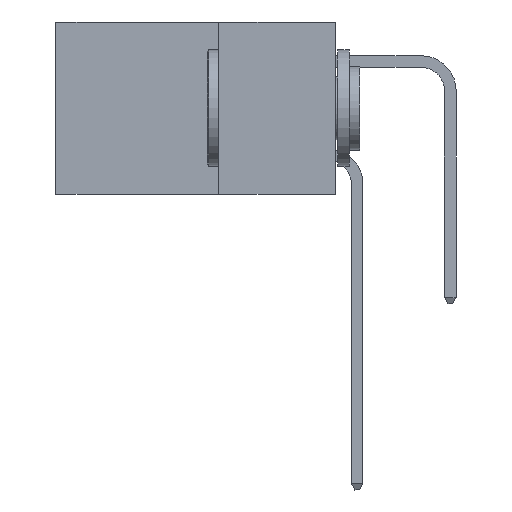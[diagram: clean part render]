
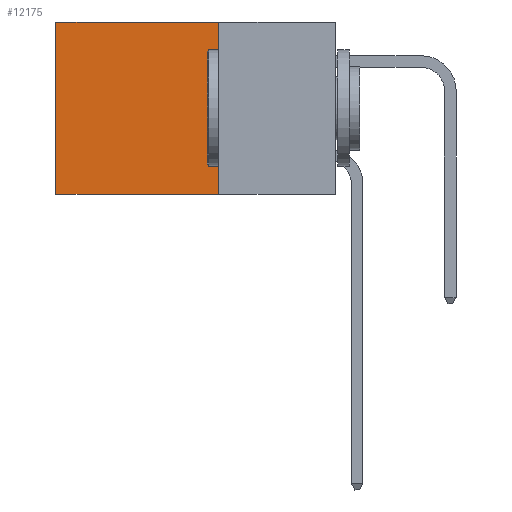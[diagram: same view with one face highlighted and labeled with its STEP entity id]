
A CAD part, left-side view. The second image highlights one B-rep face of the part: STEP entity #12175.
In plain terms, the highlighted planar face has unit normal (-1, 0, 0).
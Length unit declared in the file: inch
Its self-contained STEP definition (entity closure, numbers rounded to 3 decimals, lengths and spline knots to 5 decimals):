
#301 = VECTOR ( 'NONE', #4368, 39.37008 ) ;
#489 = VERTEX_POINT ( 'NONE', #13415 ) ;
#593 = VERTEX_POINT ( 'NONE', #12714 ) ;
#670 = FACE_OUTER_BOUND ( 'NONE', #8879, .T. ) ;
#791 = CARTESIAN_POINT ( 'NONE',  ( 0.2875, 0.25, -0.37 ) ) ;
#1101 = CARTESIAN_POINT ( 'NONE',  ( 0.2875, 0.25, 0. ) ) ;
#2113 = ORIENTED_EDGE ( 'NONE', *, *, #2717, .F. ) ;
#2717 = EDGE_CURVE ( 'NONE', #12955, #593, #13795, .T. ) ;
#2786 = DIRECTION ( 'NONE',  ( 1., 0., 0. ) ) ;
#3747 = LINE ( 'NONE', #8854, #6549 ) ;
#4368 = DIRECTION ( 'NONE',  ( 0., 1., 0. ) ) ;
#4374 = CARTESIAN_POINT ( 'NONE',  ( 0.2875, 0.25, -0.37 ) ) ;
#4686 = LINE ( 'NONE', #13721, #7107 ) ;
#4721 = VECTOR ( 'NONE', #8616, 39.37008 ) ;
#5503 = DIRECTION ( 'NONE',  ( 0., 0., -1. ) ) ;
#5987 = CARTESIAN_POINT ( 'NONE',  ( 0.2875, 0.25, 0. ) ) ;
#6377 = ORIENTED_EDGE ( 'NONE', *, *, #12557, .T. ) ;
#6549 = VECTOR ( 'NONE', #6787, 39.37008 ) ;
#6787 = DIRECTION ( 'NONE',  ( 0., 0., -1. ) ) ;
#7107 = VECTOR ( 'NONE', #5503, 39.37008 ) ;
#8616 = DIRECTION ( 'NONE',  ( 0., 1., 0. ) ) ;
#8854 = CARTESIAN_POINT ( 'NONE',  ( 0.2875, 0.6, 0. ) ) ;
#8858 = EDGE_CURVE ( 'NONE', #11644, #489, #9550, .T. ) ;
#8879 = EDGE_LOOP ( 'NONE', ( #6377, #2113, #11048, #10241 ) ) ;
#9550 = LINE ( 'NONE', #1101, #4721 ) ;
#10119 = DIRECTION ( 'NONE',  ( 0., 0., -1. ) ) ;
#10134 = EDGE_CURVE ( 'NONE', #11644, #12955, #4686, .T. ) ;
#10241 = ORIENTED_EDGE ( 'NONE', *, *, #8858, .T. ) ;
#11048 = ORIENTED_EDGE ( 'NONE', *, *, #10134, .F. ) ;
#11081 = PLANE ( 'NONE',  #13738 ) ;
#11644 = VERTEX_POINT ( 'NONE', #13297 ) ;
#12175 = ADVANCED_FACE ( 'NONE', ( #670 ), #11081, .F. ) ;
#12557 = EDGE_CURVE ( 'NONE', #489, #593, #3747, .T. ) ;
#12714 = CARTESIAN_POINT ( 'NONE',  ( 0.2875, 0.6, -0.37 ) ) ;
#12955 = VERTEX_POINT ( 'NONE', #791 ) ;
#13297 = CARTESIAN_POINT ( 'NONE',  ( 0.2875, 0.25, 0. ) ) ;
#13415 = CARTESIAN_POINT ( 'NONE',  ( 0.2875, 0.6, 0. ) ) ;
#13721 = CARTESIAN_POINT ( 'NONE',  ( 0.2875, 0.25, 0. ) ) ;
#13738 = AXIS2_PLACEMENT_3D ( 'NONE', #5987, #2786, #10119 ) ;
#13795 = LINE ( 'NONE', #4374, #301 ) ;
